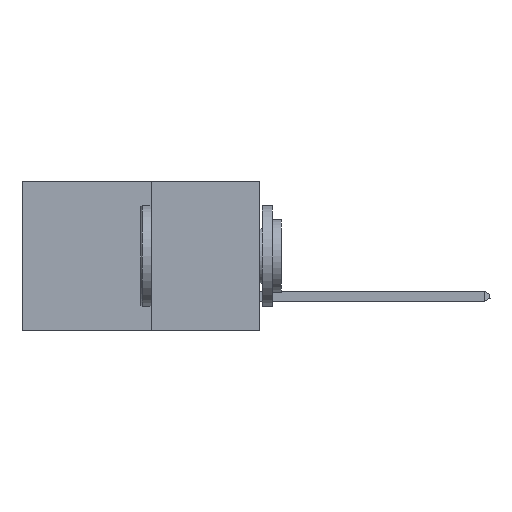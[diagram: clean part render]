
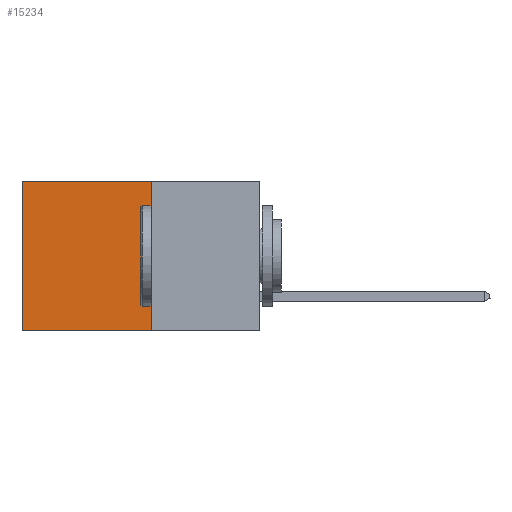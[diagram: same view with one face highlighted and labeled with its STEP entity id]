
A CAD part, left-side view. The second image highlights one B-rep face of the part: STEP entity #15234.
In plain terms, the highlighted planar face has unit normal (-1, 0, 0).
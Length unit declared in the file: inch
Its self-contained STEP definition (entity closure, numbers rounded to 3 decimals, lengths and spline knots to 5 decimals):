
#743 = FACE_OUTER_BOUND ( 'NONE', #17891, .T. ) ;
#1304 = DIRECTION ( 'NONE',  ( 0., 0., -1. ) ) ;
#1474 = DIRECTION ( 'NONE',  ( 0., 1., 0. ) ) ;
#1540 = CARTESIAN_POINT ( 'NONE',  ( 0.277, 0.27, 0. ) ) ;
#2310 = VERTEX_POINT ( 'NONE', #5617 ) ;
#2520 = LINE ( 'NONE', #17937, #20078 ) ;
#2661 = DIRECTION ( 'NONE',  ( 0., 1., 0. ) ) ;
#2678 = LINE ( 'NONE', #4573, #19186 ) ;
#4573 = CARTESIAN_POINT ( 'NONE',  ( 0.277, 0.27, -0.37 ) ) ;
#4677 = LINE ( 'NONE', #17397, #13249 ) ;
#5163 = AXIS2_PLACEMENT_3D ( 'NONE', #11601, #8248, #20169 ) ;
#5617 = CARTESIAN_POINT ( 'NONE',  ( 0.277, 0.27, 0. ) ) ;
#6638 = VERTEX_POINT ( 'NONE', #21021 ) ;
#8248 = DIRECTION ( 'NONE',  ( 1., 0., 0. ) ) ;
#8500 = EDGE_CURVE ( 'NONE', #2310, #12315, #9314, .T. ) ;
#8787 = VECTOR ( 'NONE', #1474, 39.37008 ) ;
#9314 = LINE ( 'NONE', #1540, #8787 ) ;
#9921 = VERTEX_POINT ( 'NONE', #11093 ) ;
#10668 = CARTESIAN_POINT ( 'NONE',  ( 0.277, 0.59, 0. ) ) ;
#11093 = CARTESIAN_POINT ( 'NONE',  ( 0.277, 0.59, -0.37 ) ) ;
#11360 = ORIENTED_EDGE ( 'NONE', *, *, #8500, .T. ) ;
#11601 = CARTESIAN_POINT ( 'NONE',  ( 0.277, 0.27, -0.37 ) ) ;
#12008 = EDGE_CURVE ( 'NONE', #2310, #6638, #2678, .T. ) ;
#12315 = VERTEX_POINT ( 'NONE', #10668 ) ;
#13101 = ORIENTED_EDGE ( 'NONE', *, *, #14807, .T. ) ;
#13249 = VECTOR ( 'NONE', #20766, 39.37008 ) ;
#14807 = EDGE_CURVE ( 'NONE', #12315, #9921, #4677, .T. ) ;
#15201 = ORIENTED_EDGE ( 'NONE', *, *, #12008, .F. ) ;
#15234 = ADVANCED_FACE ( 'NONE', ( #743 ), #18490, .F. ) ;
#15977 = ORIENTED_EDGE ( 'NONE', *, *, #16208, .F. ) ;
#16208 = EDGE_CURVE ( 'NONE', #6638, #9921, #2520, .T. ) ;
#17397 = CARTESIAN_POINT ( 'NONE',  ( 0.277, 0.59, -0.37 ) ) ;
#17891 = EDGE_LOOP ( 'NONE', ( #13101, #15977, #15201, #11360 ) ) ;
#17937 = CARTESIAN_POINT ( 'NONE',  ( 0.277, 0.27, -0.37 ) ) ;
#18490 = PLANE ( 'NONE',  #5163 ) ;
#19186 = VECTOR ( 'NONE', #1304, 39.37008 ) ;
#20078 = VECTOR ( 'NONE', #2661, 39.37008 ) ;
#20169 = DIRECTION ( 'NONE',  ( 0., 0., -1. ) ) ;
#20766 = DIRECTION ( 'NONE',  ( 0., 0., -1. ) ) ;
#21021 = CARTESIAN_POINT ( 'NONE',  ( 0.277, 0.27, -0.37 ) ) ;
